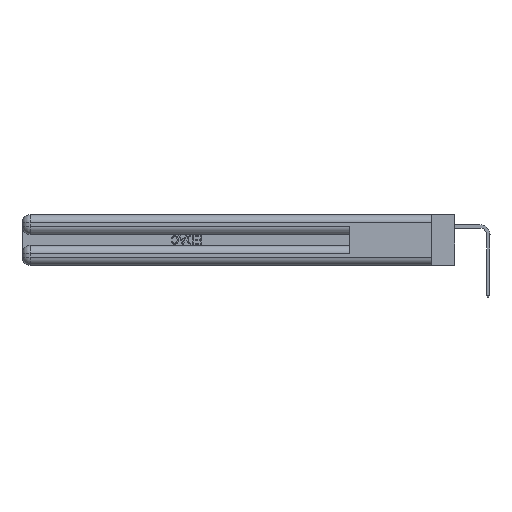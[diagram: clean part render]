
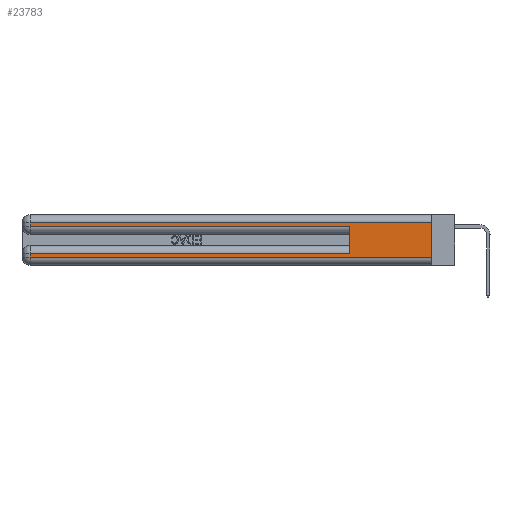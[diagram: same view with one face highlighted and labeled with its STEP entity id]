
A CAD part, left-side view. The second image highlights one B-rep face of the part: STEP entity #23783.
In plain terms, the highlighted planar face has unit normal (-1, 0, 0).
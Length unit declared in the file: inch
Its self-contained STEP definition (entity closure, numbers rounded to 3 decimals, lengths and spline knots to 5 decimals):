
#225 = CARTESIAN_POINT ( 'NONE',  ( 0., 0., 0.285 ) ) ;
#4473 = EDGE_CURVE ( 'NONE', #14962, #41931, #7931, .T. ) ;
#6841 = LINE ( 'NONE', #47429, #29616 ) ;
#7931 = LINE ( 'NONE', #20383, #52167 ) ;
#8576 = CARTESIAN_POINT ( 'NONE',  ( 0., 0., 0.06 ) ) ;
#11679 = VERTEX_POINT ( 'NONE', #44751 ) ;
#12050 = ORIENTED_EDGE ( 'NONE', *, *, #41370, .F. ) ;
#12155 = DIRECTION ( 'NONE',  ( 1., 0., 0. ) ) ;
#12679 = ORIENTED_EDGE ( 'NONE', *, *, #14828, .T. ) ;
#14142 = CARTESIAN_POINT ( 'NONE',  ( 0., 0., 0.085 ) ) ;
#14607 = CARTESIAN_POINT ( 'NONE',  ( 0., 0., 0.06 ) ) ;
#14828 = EDGE_CURVE ( 'NONE', #11679, #16207, #32392, .T. ) ;
#14962 = VERTEX_POINT ( 'NONE', #49177 ) ;
#15240 = FACE_OUTER_BOUND ( 'NONE', #49032, .T. ) ;
#16207 = VERTEX_POINT ( 'NONE', #43155 ) ;
#18389 = DIRECTION ( 'NONE',  ( 0., 1., 0. ) ) ;
#18819 = LINE ( 'NONE', #42180, #30232 ) ;
#18923 = ORIENTED_EDGE ( 'NONE', *, *, #47986, .T. ) ;
#19571 = ORIENTED_EDGE ( 'NONE', *, *, #22679, .T. ) ;
#20383 = CARTESIAN_POINT ( 'NONE',  ( 0., 0., 0.31 ) ) ;
#20922 = VECTOR ( 'NONE', #44130, 39.37008 ) ;
#21326 = LINE ( 'NONE', #28215, #31464 ) ;
#21722 = DIRECTION ( 'NONE',  ( 0., 0., -1. ) ) ;
#22679 = EDGE_CURVE ( 'NONE', #44018, #33011, #38822, .T. ) ;
#23783 = ADVANCED_FACE ( 'NONE', ( #15240 ), #33534, .F. ) ;
#25494 = CARTESIAN_POINT ( 'NONE',  ( 0., 0.6, 0.145 ) ) ;
#25934 = DIRECTION ( 'NONE',  ( 0., -1., 0. ) ) ;
#27851 = ORIENTED_EDGE ( 'NONE', *, *, #27971, .T. ) ;
#27971 = EDGE_CURVE ( 'NONE', #41931, #44018, #18819, .T. ) ;
#28215 = CARTESIAN_POINT ( 'NONE',  ( 0., 2.94, 0.37 ) ) ;
#29616 = VECTOR ( 'NONE', #21722, 39.37008 ) ;
#30039 = DIRECTION ( 'NONE',  ( 0., 0., 1. ) ) ;
#30232 = VECTOR ( 'NONE', #33596, 39.37008 ) ;
#30906 = CARTESIAN_POINT ( 'NONE',  ( 0., 2.94, 0.31 ) ) ;
#31464 = VECTOR ( 'NONE', #45292, 39.37008 ) ;
#31953 = VECTOR ( 'NONE', #38557, 39.37008 ) ;
#32392 = LINE ( 'NONE', #14142, #20922 ) ;
#33011 = VERTEX_POINT ( 'NONE', #38915 ) ;
#33534 = PLANE ( 'NONE',  #36447 ) ;
#33596 = DIRECTION ( 'NONE',  ( 0., 0., -1. ) ) ;
#34181 = ORIENTED_EDGE ( 'NONE', *, *, #39395, .F. ) ;
#36447 = AXIS2_PLACEMENT_3D ( 'NONE', #37818, #12155, #42110 ) ;
#36721 = VERTEX_POINT ( 'NONE', #53510 ) ;
#37035 = ORIENTED_EDGE ( 'NONE', *, *, #49534, .T. ) ;
#37818 = CARTESIAN_POINT ( 'NONE',  ( 0., 0., 0.37 ) ) ;
#38557 = DIRECTION ( 'NONE',  ( 0., -1., 0. ) ) ;
#38822 = LINE ( 'NONE', #225, #48892 ) ;
#38915 = CARTESIAN_POINT ( 'NONE',  ( 0., 0.6, 0.285 ) ) ;
#39395 = EDGE_CURVE ( 'NONE', #11679, #33011, #52209, .T. ) ;
#40425 = CARTESIAN_POINT ( 'NONE',  ( 0., 2.94, 0.285 ) ) ;
#40825 = VECTOR ( 'NONE', #30039, 39.37008 ) ;
#41370 = EDGE_CURVE ( 'NONE', #14962, #47398, #6841, .T. ) ;
#41931 = VERTEX_POINT ( 'NONE', #30906 ) ;
#41955 = LINE ( 'NONE', #8576, #31953 ) ;
#42110 = DIRECTION ( 'NONE',  ( 0., 0., -1. ) ) ;
#42180 = CARTESIAN_POINT ( 'NONE',  ( 0., 2.94, 0.37 ) ) ;
#43155 = CARTESIAN_POINT ( 'NONE',  ( 0., 2.94, 0.085 ) ) ;
#44018 = VERTEX_POINT ( 'NONE', #40425 ) ;
#44130 = DIRECTION ( 'NONE',  ( 0., 1., 0. ) ) ;
#44751 = CARTESIAN_POINT ( 'NONE',  ( 0., 0.6, 0.085 ) ) ;
#45292 = DIRECTION ( 'NONE',  ( 0., 0., -1. ) ) ;
#47398 = VERTEX_POINT ( 'NONE', #14607 ) ;
#47429 = CARTESIAN_POINT ( 'NONE',  ( 0., 0., 0.37 ) ) ;
#47986 = EDGE_CURVE ( 'NONE', #16207, #36721, #21326, .T. ) ;
#48755 = ORIENTED_EDGE ( 'NONE', *, *, #4473, .T. ) ;
#48892 = VECTOR ( 'NONE', #25934, 39.37008 ) ;
#49032 = EDGE_LOOP ( 'NONE', ( #12050, #48755, #27851, #19571, #34181, #12679, #18923, #37035 ) ) ;
#49177 = CARTESIAN_POINT ( 'NONE',  ( 0., 0., 0.31 ) ) ;
#49534 = EDGE_CURVE ( 'NONE', #36721, #47398, #41955, .T. ) ;
#52167 = VECTOR ( 'NONE', #18389, 39.37008 ) ;
#52209 = LINE ( 'NONE', #25494, #40825 ) ;
#53510 = CARTESIAN_POINT ( 'NONE',  ( 0., 2.94, 0.06 ) ) ;
